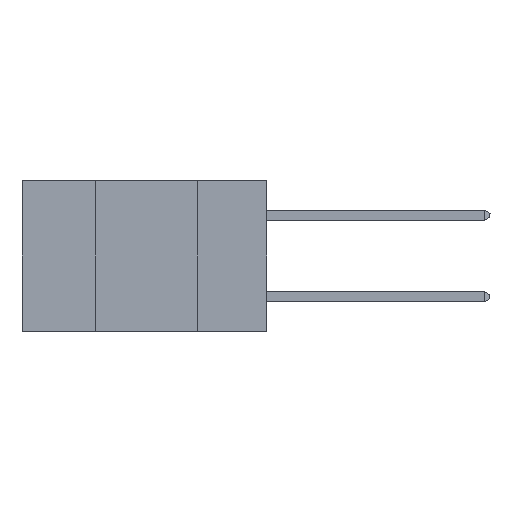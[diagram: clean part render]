
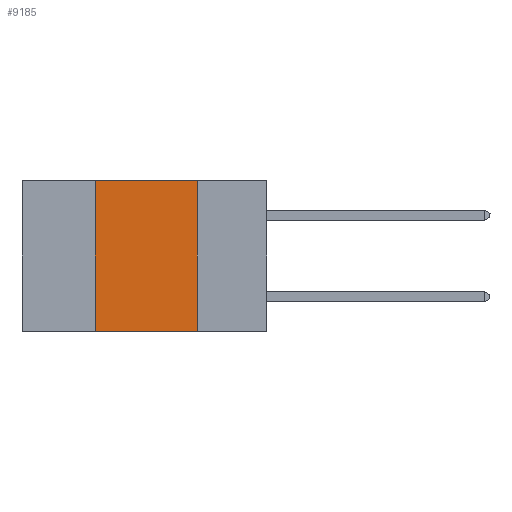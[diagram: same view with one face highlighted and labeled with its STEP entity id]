
A CAD part, left-side view. The second image highlights one B-rep face of the part: STEP entity #9185.
In plain terms, the highlighted planar face has unit normal (-1, 0, 0).
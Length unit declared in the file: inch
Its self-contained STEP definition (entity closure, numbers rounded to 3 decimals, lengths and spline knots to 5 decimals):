
#492 = VECTOR ( 'NONE', #16878, 39.37008 ) ;
#802 = CARTESIAN_POINT ( 'NONE',  ( 0., 0.42, 0. ) ) ;
#829 = CARTESIAN_POINT ( 'NONE',  ( 0., 0.42, 0. ) ) ;
#3798 = DIRECTION ( 'NONE',  ( 0., 0., -1. ) ) ;
#3819 = CARTESIAN_POINT ( 'NONE',  ( 0., 0.17, 0. ) ) ;
#4933 = CARTESIAN_POINT ( 'NONE',  ( 0., 0.42, -0.37 ) ) ;
#9185 = ADVANCED_FACE ( 'NONE', ( #26561 ), #22124, .F. ) ;
#10560 = VECTOR ( 'NONE', #16832, 39.37008 ) ;
#12701 = CARTESIAN_POINT ( 'NONE',  ( 0., 0.17, 0. ) ) ;
#14432 = DIRECTION ( 'NONE',  ( 0., -1., 0. ) ) ;
#14698 = LINE ( 'NONE', #802, #492 ) ;
#14885 = CARTESIAN_POINT ( 'NONE',  ( 0., 0.17, -0.37 ) ) ;
#15394 = EDGE_CURVE ( 'NONE', #19499, #22461, #30885, .T. ) ;
#16832 = DIRECTION ( 'NONE',  ( 0., -1., 0. ) ) ;
#16878 = DIRECTION ( 'NONE',  ( 0., 0., 1. ) ) ;
#18806 = LINE ( 'NONE', #12701, #32933 ) ;
#19499 = VERTEX_POINT ( 'NONE', #4933 ) ;
#19540 = ORIENTED_EDGE ( 'NONE', *, *, #26249, .F. ) ;
#22124 = PLANE ( 'NONE',  #26614 ) ;
#22461 = VERTEX_POINT ( 'NONE', #14885 ) ;
#22509 = CARTESIAN_POINT ( 'NONE',  ( 0., 0.6, 0. ) ) ;
#24621 = VECTOR ( 'NONE', #14432, 39.37008 ) ;
#24810 = DIRECTION ( 'NONE',  ( 1., 0., 0. ) ) ;
#24978 = CARTESIAN_POINT ( 'NONE',  ( 0., 0.6, -0.37 ) ) ;
#25044 = CARTESIAN_POINT ( 'NONE',  ( 0., 0.6, 0. ) ) ;
#25925 = EDGE_CURVE ( 'NONE', #19499, #34324, #14698, .T. ) ;
#26249 = EDGE_CURVE ( 'NONE', #32438, #22461, #18806, .T. ) ;
#26561 = FACE_OUTER_BOUND ( 'NONE', #30370, .T. ) ;
#26614 = AXIS2_PLACEMENT_3D ( 'NONE', #25044, #24810, #3798 ) ;
#27110 = ORIENTED_EDGE ( 'NONE', *, *, #25925, .F. ) ;
#27607 = LINE ( 'NONE', #22509, #10560 ) ;
#28380 = ORIENTED_EDGE ( 'NONE', *, *, #15394, .T. ) ;
#28489 = DIRECTION ( 'NONE',  ( 0., 0., -1. ) ) ;
#29527 = ORIENTED_EDGE ( 'NONE', *, *, #32478, .F. ) ;
#30370 = EDGE_LOOP ( 'NONE', ( #19540, #29527, #27110, #28380 ) ) ;
#30885 = LINE ( 'NONE', #24978, #24621 ) ;
#32438 = VERTEX_POINT ( 'NONE', #3819 ) ;
#32478 = EDGE_CURVE ( 'NONE', #34324, #32438, #27607, .T. ) ;
#32933 = VECTOR ( 'NONE', #28489, 39.37008 ) ;
#34324 = VERTEX_POINT ( 'NONE', #829 ) ;
